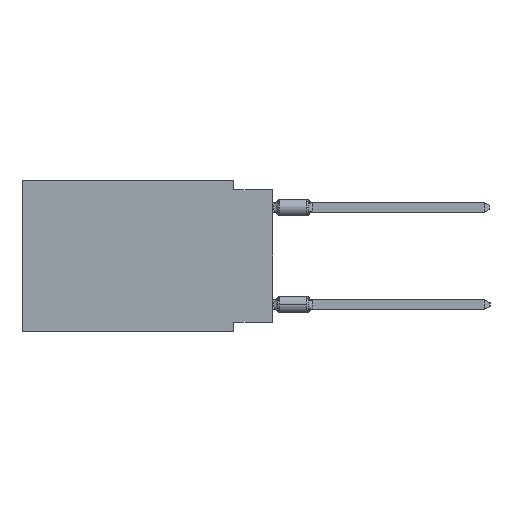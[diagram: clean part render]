
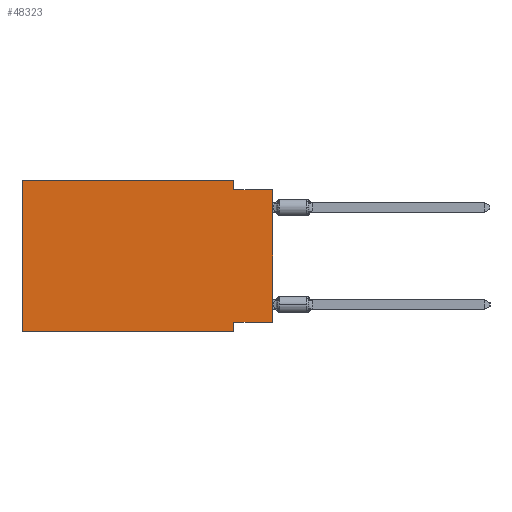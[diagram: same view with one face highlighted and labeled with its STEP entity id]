
A CAD part, left-side view. The second image highlights one B-rep face of the part: STEP entity #48323.
In plain terms, the highlighted planar face has unit normal (-1, 0, 0).
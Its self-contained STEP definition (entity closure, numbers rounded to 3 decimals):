
#530 = DIRECTION ( 'NONE',  ( 0., 0., -1. ) ) ;
#715 = EDGE_CURVE ( 'NONE', #52966, #40008, #13968, .T. ) ;
#1755 = CARTESIAN_POINT ( 'NONE',  ( 0., 2.54, -9.271 ) ) ;
#3382 = DIRECTION ( 'NONE',  ( 0., -1., 0. ) ) ;
#3552 = DIRECTION ( 'NONE',  ( 0., 0., 1. ) ) ;
#3773 = VERTEX_POINT ( 'NONE', #43435 ) ;
#4352 = EDGE_CURVE ( 'NONE', #22721, #27223, #50784, .T. ) ;
#5506 = DIRECTION ( 'NONE',  ( 1., 0., 0. ) ) ;
#6569 = CARTESIAN_POINT ( 'NONE',  ( 0., 0., -9.271 ) ) ;
#8073 = VECTOR ( 'NONE', #530, 1000. ) ;
#9462 = CARTESIAN_POINT ( 'NONE',  ( 0., 16.383, 0. ) ) ;
#10757 = CARTESIAN_POINT ( 'NONE',  ( 0., 2.54, -9.906 ) ) ;
#11355 = EDGE_CURVE ( 'NONE', #51126, #3773, #47208, .T. ) ;
#13544 = LINE ( 'NONE', #57500, #47059 ) ;
#13968 = LINE ( 'NONE', #53981, #23951 ) ;
#14399 = EDGE_CURVE ( 'NONE', #51126, #22721, #46911, .T. ) ;
#14891 = VECTOR ( 'NONE', #16320, 1000. ) ;
#16320 = DIRECTION ( 'NONE',  ( 0., 0., -1. ) ) ;
#16487 = CARTESIAN_POINT ( 'NONE',  ( 0., 0., -0.635 ) ) ;
#19622 = VECTOR ( 'NONE', #3552, 1000. ) ;
#22625 = CARTESIAN_POINT ( 'NONE',  ( 0., 16.383, -9.906 ) ) ;
#22716 = ORIENTED_EDGE ( 'NONE', *, *, #715, .F. ) ;
#22721 = VERTEX_POINT ( 'NONE', #1755 ) ;
#23951 = VECTOR ( 'NONE', #54965, 1000. ) ;
#24533 = PLANE ( 'NONE',  #40085 ) ;
#25481 = VECTOR ( 'NONE', #47319, 1000. ) ;
#25500 = DIRECTION ( 'NONE',  ( 0., 0., -1. ) ) ;
#25742 = EDGE_CURVE ( 'NONE', #29912, #45572, #55304, .T. ) ;
#26342 = ORIENTED_EDGE ( 'NONE', *, *, #25742, .F. ) ;
#27223 = VERTEX_POINT ( 'NONE', #34557 ) ;
#29750 = CARTESIAN_POINT ( 'NONE',  ( 0., 16.383, 0. ) ) ;
#29912 = VERTEX_POINT ( 'NONE', #58787 ) ;
#30678 = EDGE_CURVE ( 'NONE', #52966, #27223, #13544, .T. ) ;
#34557 = CARTESIAN_POINT ( 'NONE',  ( 0., 2.54, -9.906 ) ) ;
#34611 = CARTESIAN_POINT ( 'NONE',  ( 0., 16.383, 0. ) ) ;
#34941 = LINE ( 'NONE', #34611, #49547 ) ;
#37073 = DIRECTION ( 'NONE',  ( 0., 1., 0. ) ) ;
#40008 = VERTEX_POINT ( 'NONE', #29750 ) ;
#40085 = AXIS2_PLACEMENT_3D ( 'NONE', #9462, #5506, #25500 ) ;
#40440 = ORIENTED_EDGE ( 'NONE', *, *, #11355, .T. ) ;
#41505 = CARTESIAN_POINT ( 'NONE',  ( 0., 2.54, -0.635 ) ) ;
#43435 = CARTESIAN_POINT ( 'NONE',  ( 0., 0., -0.635 ) ) ;
#45489 = ORIENTED_EDGE ( 'NONE', *, *, #51129, .F. ) ;
#45572 = VERTEX_POINT ( 'NONE', #41505 ) ;
#46715 = EDGE_LOOP ( 'NONE', ( #40440, #45489, #26342, #49542, #22716, #53461, #50327, #56794 ) ) ;
#46911 = LINE ( 'NONE', #6569, #57496 ) ;
#47059 = VECTOR ( 'NONE', #3382, 1000. ) ;
#47208 = LINE ( 'NONE', #62906, #19622 ) ;
#47319 = DIRECTION ( 'NONE',  ( 0., -1., 0. ) ) ;
#48323 = ADVANCED_FACE ( 'NONE', ( #50455 ), #24533, .F. ) ;
#49542 = ORIENTED_EDGE ( 'NONE', *, *, #59934, .F. ) ;
#49547 = VECTOR ( 'NONE', #55890, 1000. ) ;
#50327 = ORIENTED_EDGE ( 'NONE', *, *, #4352, .F. ) ;
#50455 = FACE_OUTER_BOUND ( 'NONE', #46715, .T. ) ;
#50784 = LINE ( 'NONE', #10757, #14891 ) ;
#51126 = VERTEX_POINT ( 'NONE', #61412 ) ;
#51129 = EDGE_CURVE ( 'NONE', #45572, #3773, #62378, .T. ) ;
#52966 = VERTEX_POINT ( 'NONE', #22625 ) ;
#53461 = ORIENTED_EDGE ( 'NONE', *, *, #30678, .T. ) ;
#53981 = CARTESIAN_POINT ( 'NONE',  ( 0., 16.383, 0. ) ) ;
#54965 = DIRECTION ( 'NONE',  ( 0., 0., 1. ) ) ;
#55304 = LINE ( 'NONE', #59564, #8073 ) ;
#55890 = DIRECTION ( 'NONE',  ( 0., -1., 0. ) ) ;
#56794 = ORIENTED_EDGE ( 'NONE', *, *, #14399, .F. ) ;
#57496 = VECTOR ( 'NONE', #37073, 1000. ) ;
#57500 = CARTESIAN_POINT ( 'NONE',  ( 0., 16.383, -9.906 ) ) ;
#58787 = CARTESIAN_POINT ( 'NONE',  ( 0., 2.54, 0. ) ) ;
#59564 = CARTESIAN_POINT ( 'NONE',  ( 0., 2.54, 0. ) ) ;
#59934 = EDGE_CURVE ( 'NONE', #40008, #29912, #34941, .T. ) ;
#61412 = CARTESIAN_POINT ( 'NONE',  ( 0., 0., -9.271 ) ) ;
#62378 = LINE ( 'NONE', #16487, #25481 ) ;
#62906 = CARTESIAN_POINT ( 'NONE',  ( 0., 0., 0. ) ) ;
